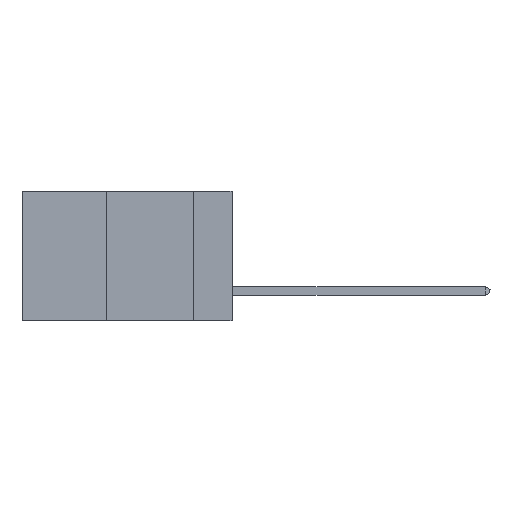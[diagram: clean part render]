
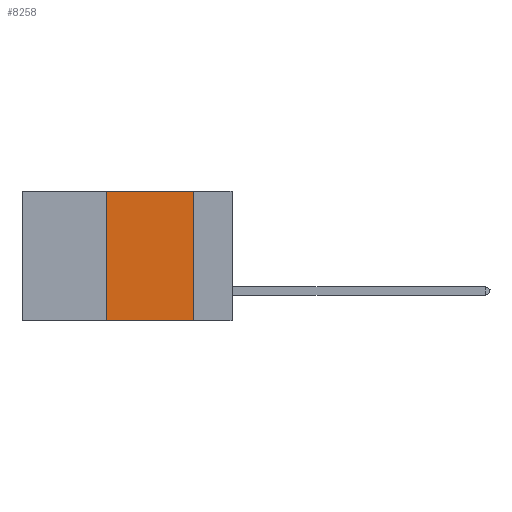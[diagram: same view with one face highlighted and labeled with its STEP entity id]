
A CAD part, left-side view. The second image highlights one B-rep face of the part: STEP entity #8258.
In plain terms, the highlighted planar face has unit normal (-1, 0, 0).
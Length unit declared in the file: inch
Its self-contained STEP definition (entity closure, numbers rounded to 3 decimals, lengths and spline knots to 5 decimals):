
#1823 = DIRECTION ( 'NONE',  ( 0., -1., 0. ) ) ;
#2288 = CARTESIAN_POINT ( 'NONE',  ( 0., 0.6, -0.37 ) ) ;
#2727 = PLANE ( 'NONE',  #34658 ) ;
#2736 = DIRECTION ( 'NONE',  ( 0., 0., 1. ) ) ;
#3439 = VECTOR ( 'NONE', #1823, 39.37008 ) ;
#4026 = DIRECTION ( 'NONE',  ( 0., 0., -1. ) ) ;
#7480 = LINE ( 'NONE', #23555, #9144 ) ;
#7636 = DIRECTION ( 'NONE',  ( 0., -1., 0. ) ) ;
#8258 = ADVANCED_FACE ( 'NONE', ( #8841 ), #2727, .F. ) ;
#8841 = FACE_OUTER_BOUND ( 'NONE', #29856, .T. ) ;
#8922 = EDGE_CURVE ( 'NONE', #18696, #30780, #17368, .T. ) ;
#9144 = VECTOR ( 'NONE', #4026, 39.37008 ) ;
#10952 = CARTESIAN_POINT ( 'NONE',  ( 0., 0.6, 0. ) ) ;
#11884 = CARTESIAN_POINT ( 'NONE',  ( 0., 0.36, -0.37 ) ) ;
#14165 = CARTESIAN_POINT ( 'NONE',  ( 0., 0.6, 0. ) ) ;
#16135 = EDGE_CURVE ( 'NONE', #18530, #18696, #32380, .T. ) ;
#17368 = LINE ( 'NONE', #10952, #29269 ) ;
#18268 = VECTOR ( 'NONE', #2736, 39.37008 ) ;
#18530 = VERTEX_POINT ( 'NONE', #11884 ) ;
#18696 = VERTEX_POINT ( 'NONE', #33617 ) ;
#19622 = LINE ( 'NONE', #2288, #3439 ) ;
#19784 = ORIENTED_EDGE ( 'NONE', *, *, #22284, .F. ) ;
#21061 = DIRECTION ( 'NONE',  ( 0., 0., -1. ) ) ;
#22284 = EDGE_CURVE ( 'NONE', #30780, #42756, #7480, .T. ) ;
#23555 = CARTESIAN_POINT ( 'NONE',  ( 0., 0.11, 0. ) ) ;
#29269 = VECTOR ( 'NONE', #7636, 39.37008 ) ;
#29856 = EDGE_LOOP ( 'NONE', ( #19784, #39426, #31481, #36277 ) ) ;
#30780 = VERTEX_POINT ( 'NONE', #32568 ) ;
#31481 = ORIENTED_EDGE ( 'NONE', *, *, #16135, .F. ) ;
#32380 = LINE ( 'NONE', #43195, #18268 ) ;
#32568 = CARTESIAN_POINT ( 'NONE',  ( 0., 0.11, 0. ) ) ;
#33617 = CARTESIAN_POINT ( 'NONE',  ( 0., 0.36, 0. ) ) ;
#34658 = AXIS2_PLACEMENT_3D ( 'NONE', #14165, #38283, #21061 ) ;
#36277 = ORIENTED_EDGE ( 'NONE', *, *, #43117, .T. ) ;
#38283 = DIRECTION ( 'NONE',  ( 1., 0., 0. ) ) ;
#39426 = ORIENTED_EDGE ( 'NONE', *, *, #8922, .F. ) ;
#42756 = VERTEX_POINT ( 'NONE', #43993 ) ;
#43117 = EDGE_CURVE ( 'NONE', #18530, #42756, #19622, .T. ) ;
#43195 = CARTESIAN_POINT ( 'NONE',  ( 0., 0.36, 0. ) ) ;
#43993 = CARTESIAN_POINT ( 'NONE',  ( 0., 0.11, -0.37 ) ) ;
